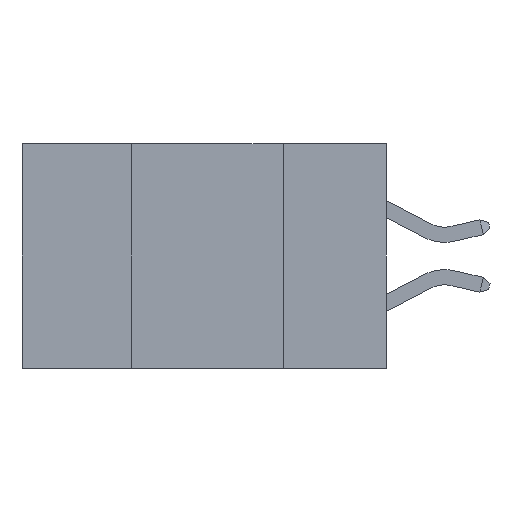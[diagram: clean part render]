
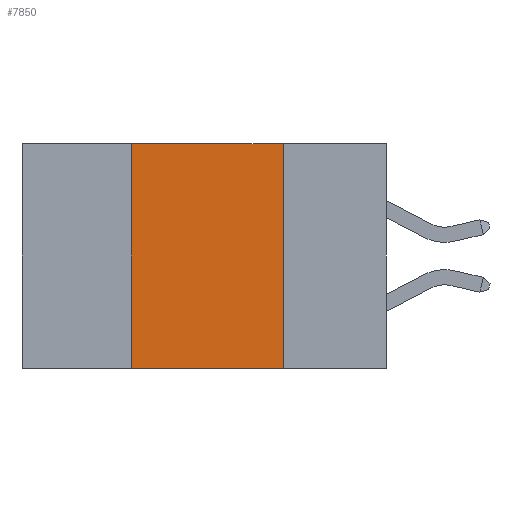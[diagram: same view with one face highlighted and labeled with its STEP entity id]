
A CAD part, left-side view. The second image highlights one B-rep face of the part: STEP entity #7850.
In plain terms, the highlighted planar face has unit normal (-1, 0, 0).
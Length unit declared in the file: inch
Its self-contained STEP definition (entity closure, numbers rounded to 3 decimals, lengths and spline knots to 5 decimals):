
#556 = LINE ( 'NONE', #11742, #11042 ) ;
#1253 = ORIENTED_EDGE ( 'NONE', *, *, #2447, .F. ) ;
#1512 = VERTEX_POINT ( 'NONE', #6105 ) ;
#1659 = ORIENTED_EDGE ( 'NONE', *, *, #2304, .F. ) ;
#2069 = EDGE_LOOP ( 'NONE', ( #4444, #1659, #1253, #6306 ) ) ;
#2125 = EDGE_CURVE ( 'NONE', #7409, #2800, #9184, .T. ) ;
#2304 = EDGE_CURVE ( 'NONE', #1512, #7409, #556, .T. ) ;
#2447 = EDGE_CURVE ( 'NONE', #9138, #1512, #7936, .T. ) ;
#2577 = EDGE_CURVE ( 'NONE', #9138, #2800, #3119, .T. ) ;
#2800 = VERTEX_POINT ( 'NONE', #12568 ) ;
#2856 = CARTESIAN_POINT ( 'NONE',  ( 0., 0.17, -0.37 ) ) ;
#3031 = DIRECTION ( 'NONE',  ( 0., 0., -1. ) ) ;
#3119 = LINE ( 'NONE', #12766, #8711 ) ;
#3319 = FACE_OUTER_BOUND ( 'NONE', #2069, .T. ) ;
#4228 = AXIS2_PLACEMENT_3D ( 'NONE', #10834, #8892, #8861 ) ;
#4444 = ORIENTED_EDGE ( 'NONE', *, *, #2125, .F. ) ;
#4829 = CARTESIAN_POINT ( 'NONE',  ( 0., 0.17, 0. ) ) ;
#6105 = CARTESIAN_POINT ( 'NONE',  ( 0., 0.42, 0. ) ) ;
#6306 = ORIENTED_EDGE ( 'NONE', *, *, #2577, .T. ) ;
#7409 = VERTEX_POINT ( 'NONE', #4829 ) ;
#7604 = VECTOR ( 'NONE', #8298, 39.37008 ) ;
#7850 = ADVANCED_FACE ( 'NONE', ( #3319 ), #8938, .F. ) ;
#7936 = LINE ( 'NONE', #8962, #7604 ) ;
#8298 = DIRECTION ( 'NONE',  ( 0., 0., 1. ) ) ;
#8711 = VECTOR ( 'NONE', #11926, 39.37008 ) ;
#8861 = DIRECTION ( 'NONE',  ( 0., 0., -1. ) ) ;
#8892 = DIRECTION ( 'NONE',  ( 1., 0., 0. ) ) ;
#8938 = PLANE ( 'NONE',  #4228 ) ;
#8962 = CARTESIAN_POINT ( 'NONE',  ( 0., 0.42, -0.37 ) ) ;
#9138 = VERTEX_POINT ( 'NONE', #10981 ) ;
#9184 = LINE ( 'NONE', #2856, #11498 ) ;
#10682 = DIRECTION ( 'NONE',  ( 0., -1., 0. ) ) ;
#10834 = CARTESIAN_POINT ( 'NONE',  ( 0., 0.6, 0. ) ) ;
#10981 = CARTESIAN_POINT ( 'NONE',  ( 0., 0.42, -0.37 ) ) ;
#11042 = VECTOR ( 'NONE', #10682, 39.37008 ) ;
#11498 = VECTOR ( 'NONE', #3031, 39.37008 ) ;
#11742 = CARTESIAN_POINT ( 'NONE',  ( 0., 0.6, 0. ) ) ;
#11926 = DIRECTION ( 'NONE',  ( 0., -1., 0. ) ) ;
#12568 = CARTESIAN_POINT ( 'NONE',  ( 0., 0.17, -0.37 ) ) ;
#12766 = CARTESIAN_POINT ( 'NONE',  ( 0., 0.6, -0.37 ) ) ;
